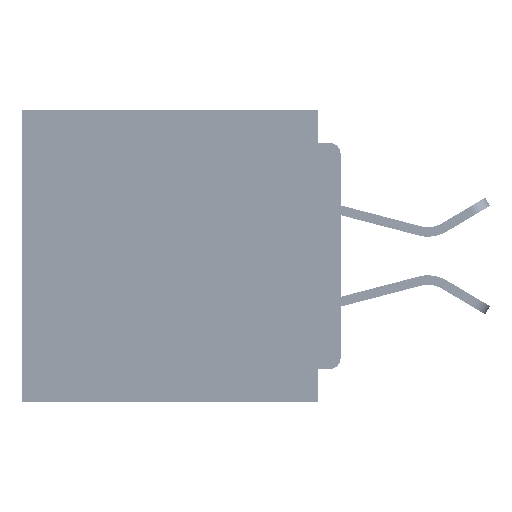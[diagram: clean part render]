
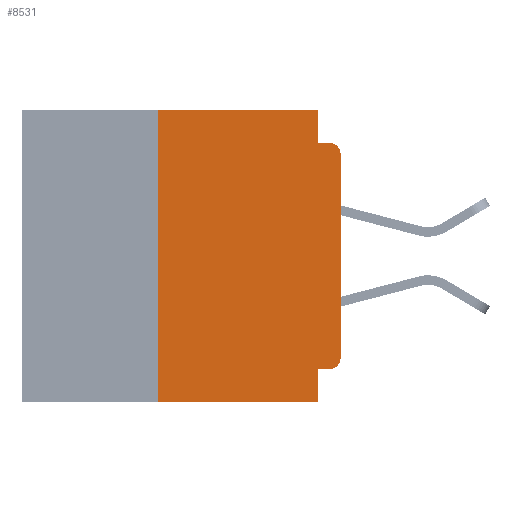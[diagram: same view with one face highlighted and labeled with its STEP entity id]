
A CAD part, left-side view. The second image highlights one B-rep face of the part: STEP entity #8531.
In plain terms, the highlighted planar face has unit normal (-1, 0, 0).
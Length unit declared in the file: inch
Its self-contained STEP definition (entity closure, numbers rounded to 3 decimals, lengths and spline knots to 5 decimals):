
#1434 = ORIENTED_EDGE ( 'NONE', *, *, #27256, .T. ) ;
#1888 = CARTESIAN_POINT ( 'NONE',  ( 0., 0.437, 0. ) ) ;
#1940 = VERTEX_POINT ( 'NONE', #5423 ) ;
#2239 = AXIS2_PLACEMENT_3D ( 'NONE', #1888, #35910, #10532 ) ;
#2879 = LINE ( 'NONE', #53818, #35450 ) ;
#3063 = VERTEX_POINT ( 'NONE', #11781 ) ;
#3544 = VERTEX_POINT ( 'NONE', #31721 ) ;
#4327 = FACE_OUTER_BOUND ( 'NONE', #12521, .T. ) ;
#4349 = EDGE_CURVE ( 'NONE', #22263, #32578, #33228, .T. ) ;
#5423 = CARTESIAN_POINT ( 'NONE',  ( 0., 0., -0.06 ) ) ;
#5714 = DIRECTION ( 'NONE',  ( 0., 0., 1. ) ) ;
#6177 = AXIS2_PLACEMENT_3D ( 'NONE', #9234, #38821, #13573 ) ;
#6406 = DIRECTION ( 'NONE',  ( 0., 1., 0. ) ) ;
#6602 = VERTEX_POINT ( 'NONE', #22489 ) ;
#6746 = CARTESIAN_POINT ( 'NONE',  ( 0., 0., -0.34 ) ) ;
#7640 = CARTESIAN_POINT ( 'NONE',  ( 0., 0.031, -0.4 ) ) ;
#7687 = DIRECTION ( 'NONE',  ( 0., 0., 1. ) ) ;
#7770 = VERTEX_POINT ( 'NONE', #17191 ) ;
#7839 = VECTOR ( 'NONE', #13202, 39.37008 ) ;
#8320 = EDGE_CURVE ( 'NONE', #1940, #32578, #25111, .T. ) ;
#8531 = ADVANCED_FACE ( 'NONE', ( #4327 ), #10348, .F. ) ;
#8857 = CARTESIAN_POINT ( 'NONE',  ( 0., 0.031, 0. ) ) ;
#9234 = CARTESIAN_POINT ( 'NONE',  ( 0., 0.015, -0.06 ) ) ;
#10016 = VECTOR ( 'NONE', #11854, 39.37008 ) ;
#10076 = CARTESIAN_POINT ( 'NONE',  ( 0., 0.015, -0.045 ) ) ;
#10348 = PLANE ( 'NONE',  #2239 ) ;
#10532 = DIRECTION ( 'NONE',  ( 0., 0., -1. ) ) ;
#10746 = CARTESIAN_POINT ( 'NONE',  ( 0., 0., -0.355 ) ) ;
#11672 = CARTESIAN_POINT ( 'NONE',  ( 0., 0.015, -0.34 ) ) ;
#11781 = CARTESIAN_POINT ( 'NONE',  ( 0., 0.25, 0. ) ) ;
#11854 = DIRECTION ( 'NONE',  ( 0., -1., 0. ) ) ;
#12521 = EDGE_LOOP ( 'NONE', ( #1434, #23037, #33657, #39474, #54648, #27711, #31219, #29940, #49781, #15256 ) ) ;
#13202 = DIRECTION ( 'NONE',  ( 0., 0., -1. ) ) ;
#13517 = VECTOR ( 'NONE', #6406, 39.37008 ) ;
#13573 = DIRECTION ( 'NONE',  ( 0., 0., -1. ) ) ;
#14204 = CARTESIAN_POINT ( 'NONE',  ( 0., 0.25, -0.4 ) ) ;
#14412 = VERTEX_POINT ( 'NONE', #37881 ) ;
#14967 = DIRECTION ( 'NONE',  ( 0., -1., 0. ) ) ;
#15256 = ORIENTED_EDGE ( 'NONE', *, *, #54439, .T. ) ;
#15589 = CARTESIAN_POINT ( 'NONE',  ( 0., 0., -0.045 ) ) ;
#15923 = VECTOR ( 'NONE', #37459, 39.37008 ) ;
#16001 = DIRECTION ( 'NONE',  ( 0., 0., -1. ) ) ;
#17191 = CARTESIAN_POINT ( 'NONE',  ( 0., 0.25, -0.4 ) ) ;
#21542 = EDGE_CURVE ( 'NONE', #3544, #49136, #38285, .T. ) ;
#21600 = VECTOR ( 'NONE', #14967, 39.37008 ) ;
#22263 = VERTEX_POINT ( 'NONE', #54422 ) ;
#22489 = CARTESIAN_POINT ( 'NONE',  ( 0., 0.015, -0.355 ) ) ;
#22940 = LINE ( 'NONE', #27743, #21600 ) ;
#23037 = ORIENTED_EDGE ( 'NONE', *, *, #8320, .T. ) ;
#25111 = CIRCLE ( 'NONE', #6177, 0.015 ) ;
#27256 = EDGE_CURVE ( 'NONE', #51836, #1940, #2879, .T. ) ;
#27280 = AXIS2_PLACEMENT_3D ( 'NONE', #11672, #41141, #16001 ) ;
#27437 = CIRCLE ( 'NONE', #27280, 0.015 ) ;
#27711 = ORIENTED_EDGE ( 'NONE', *, *, #38383, .F. ) ;
#27743 = CARTESIAN_POINT ( 'NONE',  ( 0., 0.437, 0. ) ) ;
#28316 = EDGE_CURVE ( 'NONE', #6602, #3544, #38589, .T. ) ;
#29940 = ORIENTED_EDGE ( 'NONE', *, *, #21542, .F. ) ;
#31219 = ORIENTED_EDGE ( 'NONE', *, *, #35602, .T. ) ;
#31295 = LINE ( 'NONE', #41313, #10016 ) ;
#31721 = CARTESIAN_POINT ( 'NONE',  ( 0., 0.031, -0.355 ) ) ;
#31905 = VECTOR ( 'NONE', #44925, 39.37008 ) ;
#32578 = VERTEX_POINT ( 'NONE', #10076 ) ;
#33228 = LINE ( 'NONE', #15589, #31905 ) ;
#33657 = ORIENTED_EDGE ( 'NONE', *, *, #4349, .F. ) ;
#34300 = EDGE_CURVE ( 'NONE', #3063, #14412, #22940, .T. ) ;
#35450 = VECTOR ( 'NONE', #7687, 39.37008 ) ;
#35602 = EDGE_CURVE ( 'NONE', #7770, #49136, #31295, .T. ) ;
#35910 = DIRECTION ( 'NONE',  ( 1., 0., 0. ) ) ;
#37459 = DIRECTION ( 'NONE',  ( 0., 0., -1. ) ) ;
#37881 = CARTESIAN_POINT ( 'NONE',  ( 0., 0.031, 0. ) ) ;
#38285 = LINE ( 'NONE', #7640, #15923 ) ;
#38383 = EDGE_CURVE ( 'NONE', #7770, #3063, #42513, .T. ) ;
#38589 = LINE ( 'NONE', #10746, #13517 ) ;
#38821 = DIRECTION ( 'NONE',  ( -1., 0., 0. ) ) ;
#39474 = ORIENTED_EDGE ( 'NONE', *, *, #41169, .F. ) ;
#41141 = DIRECTION ( 'NONE',  ( -1., 0., 0. ) ) ;
#41169 = EDGE_CURVE ( 'NONE', #14412, #22263, #41533, .T. ) ;
#41218 = VECTOR ( 'NONE', #5714, 39.37008 ) ;
#41313 = CARTESIAN_POINT ( 'NONE',  ( 0., 0.437, -0.4 ) ) ;
#41533 = LINE ( 'NONE', #8857, #7839 ) ;
#42513 = LINE ( 'NONE', #14204, #41218 ) ;
#44925 = DIRECTION ( 'NONE',  ( 0., -1., 0. ) ) ;
#49136 = VERTEX_POINT ( 'NONE', #54497 ) ;
#49781 = ORIENTED_EDGE ( 'NONE', *, *, #28316, .F. ) ;
#51836 = VERTEX_POINT ( 'NONE', #6746 ) ;
#53818 = CARTESIAN_POINT ( 'NONE',  ( 0., 0., 0. ) ) ;
#54422 = CARTESIAN_POINT ( 'NONE',  ( 0., 0.031, -0.045 ) ) ;
#54439 = EDGE_CURVE ( 'NONE', #6602, #51836, #27437, .T. ) ;
#54497 = CARTESIAN_POINT ( 'NONE',  ( 0., 0.031, -0.4 ) ) ;
#54648 = ORIENTED_EDGE ( 'NONE', *, *, #34300, .F. ) ;
